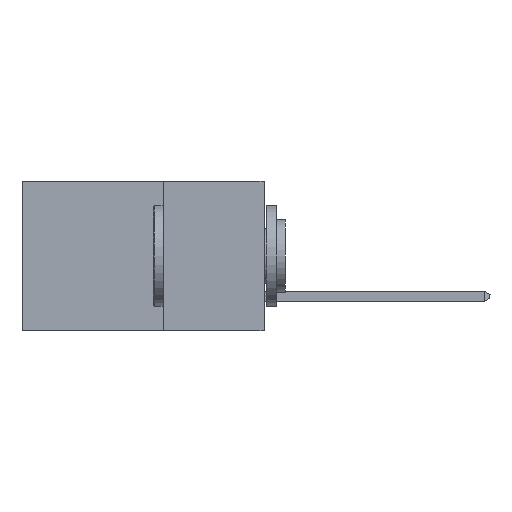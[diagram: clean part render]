
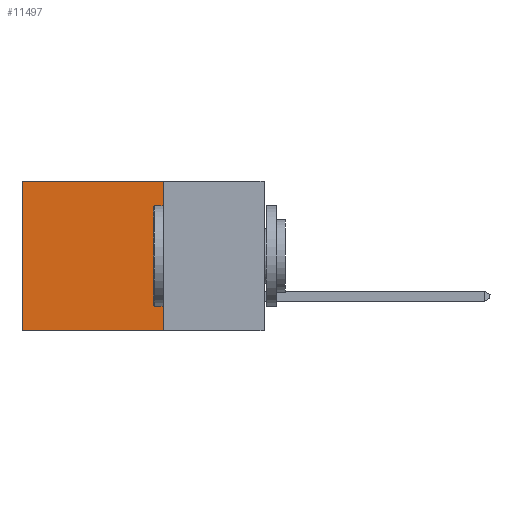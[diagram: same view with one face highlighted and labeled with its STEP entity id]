
A CAD part, left-side view. The second image highlights one B-rep face of the part: STEP entity #11497.
In plain terms, the highlighted planar face has unit normal (-1, 0, 0).
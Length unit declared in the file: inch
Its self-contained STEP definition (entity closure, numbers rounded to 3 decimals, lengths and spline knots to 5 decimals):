
#1267 = ORIENTED_EDGE ( 'NONE', *, *, #5385, .F. ) ;
#1572 = LINE ( 'NONE', #2865, #24620 ) ;
#2865 = CARTESIAN_POINT ( 'NONE',  ( 0.298, 0.25, 0. ) ) ;
#4648 = CARTESIAN_POINT ( 'NONE',  ( 0.298, 0.6, 0. ) ) ;
#5096 = FACE_OUTER_BOUND ( 'NONE', #24000, .T. ) ;
#5251 = DIRECTION ( 'NONE',  ( 1., 0., 0. ) ) ;
#5385 = EDGE_CURVE ( 'NONE', #15627, #10223, #6923, .T. ) ;
#6146 = ORIENTED_EDGE ( 'NONE', *, *, #20273, .T. ) ;
#6923 = LINE ( 'NONE', #10801, #9978 ) ;
#8372 = VECTOR ( 'NONE', #12986, 39.37008 ) ;
#8958 = DIRECTION ( 'NONE',  ( 0., 0., -1. ) ) ;
#9096 = PLANE ( 'NONE',  #16225 ) ;
#9978 = VECTOR ( 'NONE', #8958, 39.37008 ) ;
#10048 = CARTESIAN_POINT ( 'NONE',  ( 0.298, 0.25, -0.37 ) ) ;
#10223 = VERTEX_POINT ( 'NONE', #10048 ) ;
#10801 = CARTESIAN_POINT ( 'NONE',  ( 0.298, 0.25, 0. ) ) ;
#11497 = ADVANCED_FACE ( 'NONE', ( #5096 ), #9096, .F. ) ;
#12986 = DIRECTION ( 'NONE',  ( 0., 1., 0. ) ) ;
#14268 = ORIENTED_EDGE ( 'NONE', *, *, #21093, .F. ) ;
#14309 = DIRECTION ( 'NONE',  ( 0., 1., 0. ) ) ;
#15627 = VERTEX_POINT ( 'NONE', #22093 ) ;
#16225 = AXIS2_PLACEMENT_3D ( 'NONE', #16568, #5251, #20794 ) ;
#16568 = CARTESIAN_POINT ( 'NONE',  ( 0.298, 0.25, 0. ) ) ;
#17642 = CARTESIAN_POINT ( 'NONE',  ( 0.298, 0.6, 0. ) ) ;
#18123 = LINE ( 'NONE', #17642, #20222 ) ;
#18762 = CARTESIAN_POINT ( 'NONE',  ( 0.298, 0.25, -0.37 ) ) ;
#19122 = ORIENTED_EDGE ( 'NONE', *, *, #24093, .T. ) ;
#19740 = DIRECTION ( 'NONE',  ( 0., 0., -1. ) ) ;
#20222 = VECTOR ( 'NONE', #19740, 39.37008 ) ;
#20273 = EDGE_CURVE ( 'NONE', #24494, #23269, #18123, .T. ) ;
#20794 = DIRECTION ( 'NONE',  ( 0., 0., -1. ) ) ;
#21093 = EDGE_CURVE ( 'NONE', #10223, #23269, #24480, .T. ) ;
#22093 = CARTESIAN_POINT ( 'NONE',  ( 0.298, 0.25, 0. ) ) ;
#23269 = VERTEX_POINT ( 'NONE', #23380 ) ;
#23380 = CARTESIAN_POINT ( 'NONE',  ( 0.298, 0.6, -0.37 ) ) ;
#24000 = EDGE_LOOP ( 'NONE', ( #6146, #14268, #1267, #19122 ) ) ;
#24093 = EDGE_CURVE ( 'NONE', #15627, #24494, #1572, .T. ) ;
#24480 = LINE ( 'NONE', #18762, #8372 ) ;
#24494 = VERTEX_POINT ( 'NONE', #4648 ) ;
#24620 = VECTOR ( 'NONE', #14309, 39.37008 ) ;
